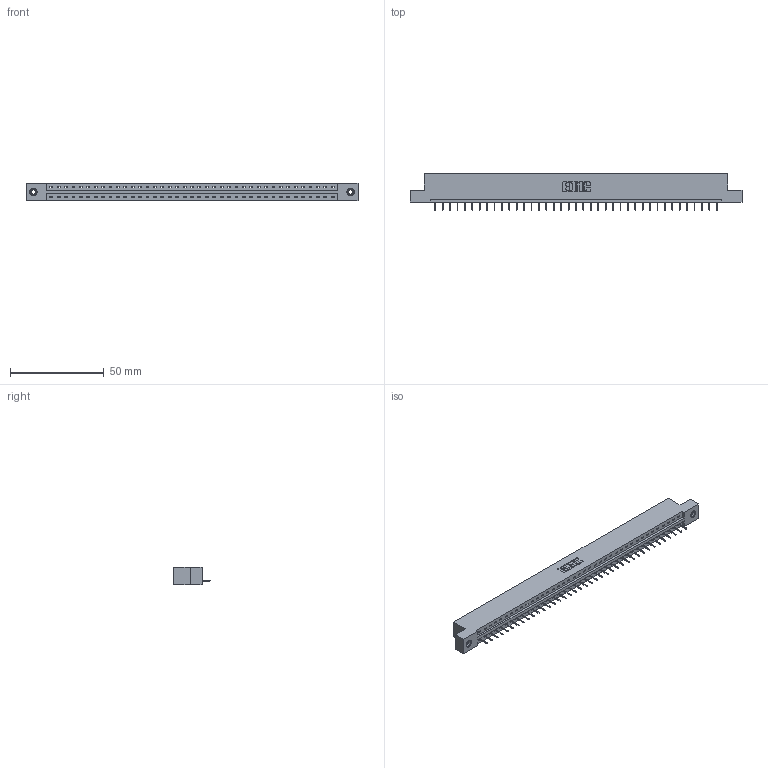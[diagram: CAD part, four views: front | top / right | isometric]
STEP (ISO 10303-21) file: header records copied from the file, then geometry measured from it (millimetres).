
FILE_DESCRIPTION (( 'STEP AP203' ), '1' );
FILE_NAME ('337-039-524-108.STEP', '2018-08-08T07:13:52', ( '' ), ( '' ), 'SwSTEP 2.0', 'SolidWorks 2016', '' );
FILE_SCHEMA (( 'CONFIG_CONTROL_DESIGN' ));
Length unit declared in the file: inch
Products named in the file (4): 337-039-524-108; 337 Part_Flush Mounting Lugs - 0.156 Dia-TI; 345-292-001_345-293-124; 345-250-001_345-250-003-102
Assembly tree (42 placements, depth 2):
  337-039-524-108
    337 Part_Flush Mounting Lugs - 0.156 Dia-TI
    345-292-001_345-293-124  x39
    345-250-001_345-250-003-102  x2
Bounding box: 177.55 x 19.69 x 9.4 mm (x, y, z)
Volume: 18254.8 mm3; surface area: 18334.9 mm2
Topology: 42 solids, 42 shells, 2748 faces, 7935 edges, 5126 vertices
Faces by surface type: plane 2130, cylinder 602, cone 12, torus 4
Entity records: 30638 total; most frequent: CARTESIAN_POINT 5314, ORIENTED_EDGE 5282, DIRECTION 4513, EDGE_CURVE 2641, LINE 2497, VECTOR 2497, VERTEX_POINT 1752, AXIS2_PLACEMENT_3D 1008
